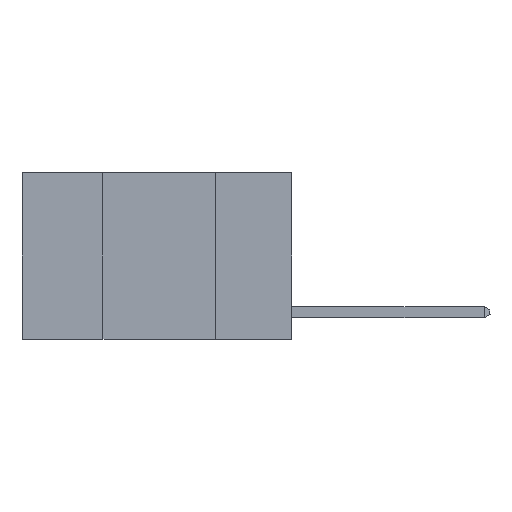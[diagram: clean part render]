
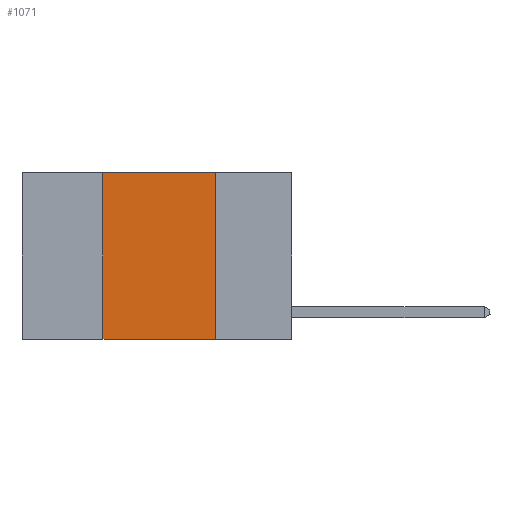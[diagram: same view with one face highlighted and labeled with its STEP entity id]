
A CAD part, left-side view. The second image highlights one B-rep face of the part: STEP entity #1071.
In plain terms, the highlighted planar face has unit normal (-1, 0, 0).
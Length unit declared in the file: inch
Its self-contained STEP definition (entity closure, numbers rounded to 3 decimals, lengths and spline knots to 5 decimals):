
#566 = CARTESIAN_POINT ( 'NONE',  ( 0., 0.17, 0. ) ) ;
#846 = PLANE ( 'NONE',  #3952 ) ;
#1071 = ADVANCED_FACE ( 'NONE', ( #2770 ), #846, .F. ) ;
#1284 = ORIENTED_EDGE ( 'NONE', *, *, #10960, .F. ) ;
#1323 = VERTEX_POINT ( 'NONE', #6488 ) ;
#1481 = LINE ( 'NONE', #5635, #6515 ) ;
#1616 = DIRECTION ( 'NONE',  ( 0., -1., 0. ) ) ;
#2331 = ORIENTED_EDGE ( 'NONE', *, *, #8493, .T. ) ;
#2770 = FACE_OUTER_BOUND ( 'NONE', #8023, .T. ) ;
#2780 = VERTEX_POINT ( 'NONE', #11512 ) ;
#2882 = LINE ( 'NONE', #7975, #6353 ) ;
#2982 = VERTEX_POINT ( 'NONE', #13123 ) ;
#3952 = AXIS2_PLACEMENT_3D ( 'NONE', #5025, #9190, #13357 ) ;
#4682 = EDGE_CURVE ( 'NONE', #2780, #1323, #5331, .T. ) ;
#4840 = LINE ( 'NONE', #7063, #13504 ) ;
#5002 = VERTEX_POINT ( 'NONE', #566 ) ;
#5025 = CARTESIAN_POINT ( 'NONE',  ( 0., 0.6, 0. ) ) ;
#5331 = LINE ( 'NONE', #8183, #8238 ) ;
#5635 = CARTESIAN_POINT ( 'NONE',  ( 0., 0.6, -0.37 ) ) ;
#6291 = EDGE_CURVE ( 'NONE', #1323, #5002, #4840, .T. ) ;
#6353 = VECTOR ( 'NONE', #7021, 39.37008 ) ;
#6488 = CARTESIAN_POINT ( 'NONE',  ( 0., 0.42, 0. ) ) ;
#6515 = VECTOR ( 'NONE', #1616, 39.37008 ) ;
#7021 = DIRECTION ( 'NONE',  ( 0., 0., -1. ) ) ;
#7063 = CARTESIAN_POINT ( 'NONE',  ( 0., 0.6, 0. ) ) ;
#7975 = CARTESIAN_POINT ( 'NONE',  ( 0., 0.17, 0. ) ) ;
#8023 = EDGE_LOOP ( 'NONE', ( #1284, #13219, #9591, #2331 ) ) ;
#8183 = CARTESIAN_POINT ( 'NONE',  ( 0., 0.42, 0. ) ) ;
#8238 = VECTOR ( 'NONE', #10432, 39.37008 ) ;
#8493 = EDGE_CURVE ( 'NONE', #2780, #2982, #1481, .T. ) ;
#9190 = DIRECTION ( 'NONE',  ( 1., 0., 0. ) ) ;
#9591 = ORIENTED_EDGE ( 'NONE', *, *, #4682, .F. ) ;
#10158 = DIRECTION ( 'NONE',  ( 0., -1., 0. ) ) ;
#10432 = DIRECTION ( 'NONE',  ( 0., 0., 1. ) ) ;
#10960 = EDGE_CURVE ( 'NONE', #5002, #2982, #2882, .T. ) ;
#11512 = CARTESIAN_POINT ( 'NONE',  ( 0., 0.42, -0.37 ) ) ;
#13123 = CARTESIAN_POINT ( 'NONE',  ( 0., 0.17, -0.37 ) ) ;
#13219 = ORIENTED_EDGE ( 'NONE', *, *, #6291, .F. ) ;
#13357 = DIRECTION ( 'NONE',  ( 0., 0., -1. ) ) ;
#13504 = VECTOR ( 'NONE', #10158, 39.37008 ) ;
